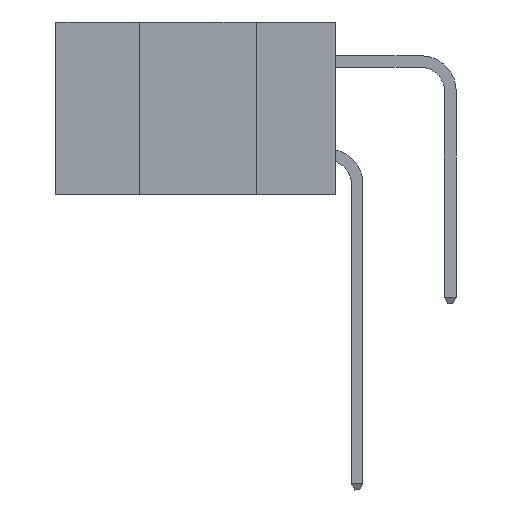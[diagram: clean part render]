
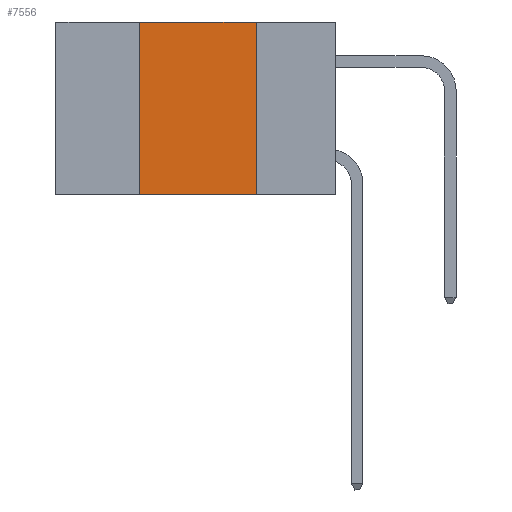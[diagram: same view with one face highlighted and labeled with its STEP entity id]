
A CAD part, left-side view. The second image highlights one B-rep face of the part: STEP entity #7556.
In plain terms, the highlighted planar face has unit normal (-1, 0, 0).
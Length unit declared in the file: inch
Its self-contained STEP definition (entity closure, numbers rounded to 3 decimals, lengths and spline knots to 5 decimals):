
#1089 = VERTEX_POINT ( 'NONE', #25373 ) ;
#3315 = VECTOR ( 'NONE', #18994, 39.37008 ) ;
#3617 = VERTEX_POINT ( 'NONE', #8490 ) ;
#4631 = CARTESIAN_POINT ( 'NONE',  ( 0., 0.17, 0. ) ) ;
#4948 = ORIENTED_EDGE ( 'NONE', *, *, #31931, .F. ) ;
#5194 = PLANE ( 'NONE',  #27181 ) ;
#6043 = VERTEX_POINT ( 'NONE', #18545 ) ;
#7556 = ADVANCED_FACE ( 'NONE', ( #20845 ), #5194, .F. ) ;
#7605 = ORIENTED_EDGE ( 'NONE', *, *, #15648, .F. ) ;
#8490 = CARTESIAN_POINT ( 'NONE',  ( 0., 0.17, -0.37 ) ) ;
#8634 = LINE ( 'NONE', #4631, #21500 ) ;
#8768 = VERTEX_POINT ( 'NONE', #23866 ) ;
#8993 = ORIENTED_EDGE ( 'NONE', *, *, #15148, .T. ) ;
#10175 = EDGE_CURVE ( 'NONE', #6043, #8768, #10368, .T. ) ;
#10368 = LINE ( 'NONE', #24185, #14811 ) ;
#11214 = CARTESIAN_POINT ( 'NONE',  ( 0., 0.42, 0. ) ) ;
#11277 = VECTOR ( 'NONE', #32876, 39.37008 ) ;
#13260 = LINE ( 'NONE', #17684, #11277 ) ;
#14811 = VECTOR ( 'NONE', #22161, 39.37008 ) ;
#15148 = EDGE_CURVE ( 'NONE', #1089, #3617, #13260, .T. ) ;
#15648 = EDGE_CURVE ( 'NONE', #1089, #6043, #30689, .T. ) ;
#15976 = ORIENTED_EDGE ( 'NONE', *, *, #10175, .F. ) ;
#17684 = CARTESIAN_POINT ( 'NONE',  ( 0., 0.6, -0.37 ) ) ;
#18474 = CARTESIAN_POINT ( 'NONE',  ( 0., 0.6, 0. ) ) ;
#18545 = CARTESIAN_POINT ( 'NONE',  ( 0., 0.42, 0. ) ) ;
#18994 = DIRECTION ( 'NONE',  ( 0., 0., 1. ) ) ;
#20845 = FACE_OUTER_BOUND ( 'NONE', #27544, .T. ) ;
#21500 = VECTOR ( 'NONE', #27724, 39.37008 ) ;
#22161 = DIRECTION ( 'NONE',  ( 0., -1., 0. ) ) ;
#23866 = CARTESIAN_POINT ( 'NONE',  ( 0., 0.17, 0. ) ) ;
#24185 = CARTESIAN_POINT ( 'NONE',  ( 0., 0.6, 0. ) ) ;
#25373 = CARTESIAN_POINT ( 'NONE',  ( 0., 0.42, -0.37 ) ) ;
#25882 = DIRECTION ( 'NONE',  ( 1., 0., 0. ) ) ;
#27181 = AXIS2_PLACEMENT_3D ( 'NONE', #18474, #25882, #30871 ) ;
#27544 = EDGE_LOOP ( 'NONE', ( #4948, #15976, #7605, #8993 ) ) ;
#27724 = DIRECTION ( 'NONE',  ( 0., 0., -1. ) ) ;
#30689 = LINE ( 'NONE', #11214, #3315 ) ;
#30871 = DIRECTION ( 'NONE',  ( 0., 0., -1. ) ) ;
#31931 = EDGE_CURVE ( 'NONE', #8768, #3617, #8634, .T. ) ;
#32876 = DIRECTION ( 'NONE',  ( 0., -1., 0. ) ) ;
